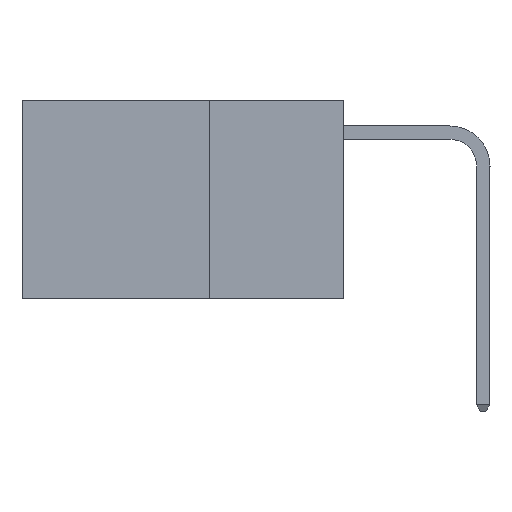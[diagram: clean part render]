
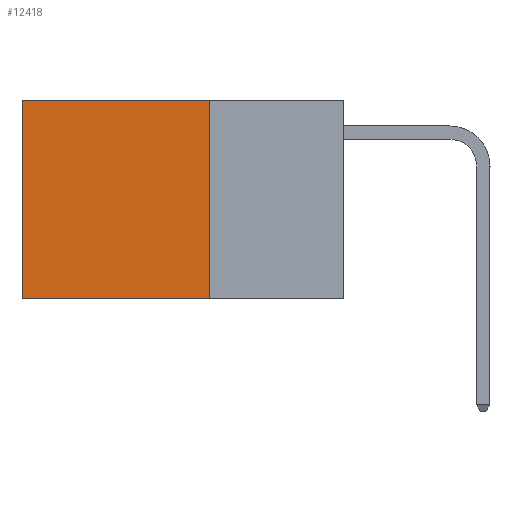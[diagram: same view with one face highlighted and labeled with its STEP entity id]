
A CAD part, left-side view. The second image highlights one B-rep face of the part: STEP entity #12418.
In plain terms, the highlighted planar face has unit normal (-1, 0, 0).
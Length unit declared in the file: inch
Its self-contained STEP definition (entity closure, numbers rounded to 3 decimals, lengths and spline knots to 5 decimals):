
#380 = VERTEX_POINT ( 'NONE', #4694 ) ;
#792 = CARTESIAN_POINT ( 'NONE',  ( 0.2625, 0.6, 0. ) ) ;
#1950 = FACE_OUTER_BOUND ( 'NONE', #17947, .T. ) ;
#3273 = ORIENTED_EDGE ( 'NONE', *, *, #12361, .F. ) ;
#3388 = CARTESIAN_POINT ( 'NONE',  ( 0.2625, 0.6, 0. ) ) ;
#3896 = CARTESIAN_POINT ( 'NONE',  ( 0.2625, 0.25, 0. ) ) ;
#4330 = LINE ( 'NONE', #792, #12584 ) ;
#4694 = CARTESIAN_POINT ( 'NONE',  ( 0.2625, 0.25, 0. ) ) ;
#5181 = VERTEX_POINT ( 'NONE', #8666 ) ;
#5576 = DIRECTION ( 'NONE',  ( 0., 0., -1. ) ) ;
#6435 = ORIENTED_EDGE ( 'NONE', *, *, #7877, .F. ) ;
#7877 = EDGE_CURVE ( 'NONE', #5181, #20858, #17724, .T. ) ;
#8666 = CARTESIAN_POINT ( 'NONE',  ( 0.2625, 0.25, -0.37 ) ) ;
#8706 = CARTESIAN_POINT ( 'NONE',  ( 0.2625, 0.25, 0. ) ) ;
#9977 = ORIENTED_EDGE ( 'NONE', *, *, #10251, .T. ) ;
#10251 = EDGE_CURVE ( 'NONE', #380, #14224, #18713, .T. ) ;
#10782 = DIRECTION ( 'NONE',  ( 0., 0., -1. ) ) ;
#11469 = DIRECTION ( 'NONE',  ( 0., 1., 0. ) ) ;
#11487 = CARTESIAN_POINT ( 'NONE',  ( 0.2625, 0.25, -0.37 ) ) ;
#11955 = CARTESIAN_POINT ( 'NONE',  ( 0.2625, 0.25, 0. ) ) ;
#12361 = EDGE_CURVE ( 'NONE', #380, #5181, #16166, .T. ) ;
#12418 = ADVANCED_FACE ( 'NONE', ( #1950 ), #13804, .F. ) ;
#12520 = EDGE_CURVE ( 'NONE', #14224, #20858, #4330, .T. ) ;
#12584 = VECTOR ( 'NONE', #10782, 39.37008 ) ;
#13614 = DIRECTION ( 'NONE',  ( 0., 1., 0. ) ) ;
#13662 = DIRECTION ( 'NONE',  ( 0., 0., -1. ) ) ;
#13804 = PLANE ( 'NONE',  #17928 ) ;
#13972 = VECTOR ( 'NONE', #11469, 39.37008 ) ;
#14224 = VERTEX_POINT ( 'NONE', #3388 ) ;
#14497 = VECTOR ( 'NONE', #13614, 39.37008 ) ;
#15460 = DIRECTION ( 'NONE',  ( 1., 0., 0. ) ) ;
#16166 = LINE ( 'NONE', #8706, #20944 ) ;
#17186 = CARTESIAN_POINT ( 'NONE',  ( 0.2625, 0.6, -0.37 ) ) ;
#17724 = LINE ( 'NONE', #11487, #13972 ) ;
#17819 = ORIENTED_EDGE ( 'NONE', *, *, #12520, .T. ) ;
#17928 = AXIS2_PLACEMENT_3D ( 'NONE', #3896, #15460, #5576 ) ;
#17947 = EDGE_LOOP ( 'NONE', ( #17819, #6435, #3273, #9977 ) ) ;
#18713 = LINE ( 'NONE', #11955, #14497 ) ;
#20858 = VERTEX_POINT ( 'NONE', #17186 ) ;
#20944 = VECTOR ( 'NONE', #13662, 39.37008 ) ;
